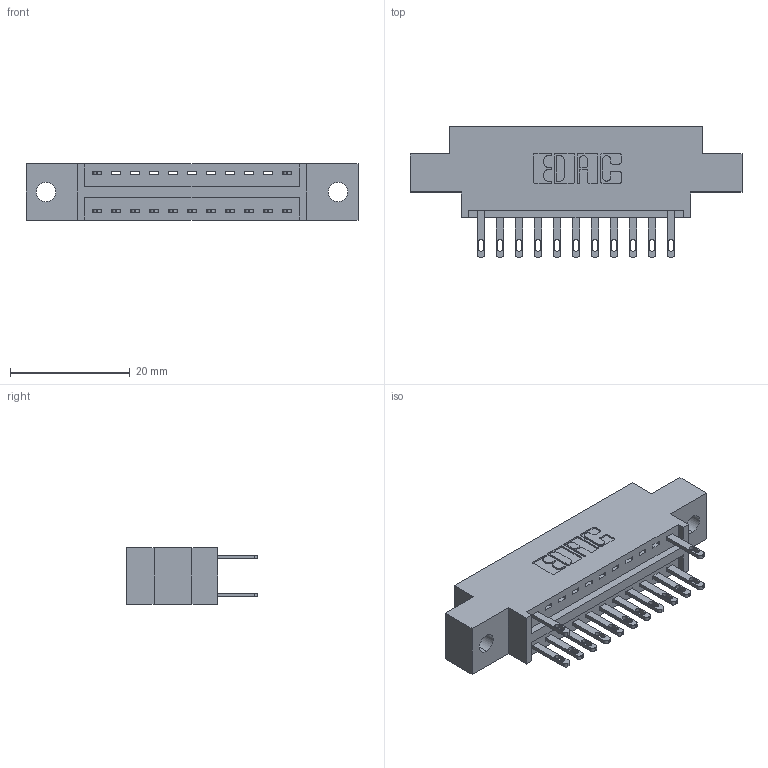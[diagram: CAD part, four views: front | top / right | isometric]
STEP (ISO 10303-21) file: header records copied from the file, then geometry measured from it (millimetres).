
FILE_DESCRIPTION (( 'STEP AP203' ), '1' );
FILE_NAME ('346-022-500-802.STEP', '2018-08-20T23:35:04', ( '' ), ( '' ), 'SwSTEP 2.0', 'SolidWorks 2016', '' );
FILE_SCHEMA (( 'CONFIG_CONTROL_DESIGN' ));
Length unit declared in the file: inch
Products named in the file (3): 345-292-001_345-293-100; 346-022-500-802; 346 Part_0.170 Offset - 0.128 Dia
Assembly tree (14 placements, depth 2):
  346-022-500-802
    346 Part_0.170 Offset - 0.128 Dia
    345-292-001_345-293-100  x13
Bounding box: 55.5 x 21.84 x 9.4 mm (x, y, z)
Volume: 4938.5 mm3; surface area: 5880.4 mm2
Topology: 14 solids, 14 shells, 804 faces, 2441 edges, 1626 vertices
Faces by surface type: plane 502, cylinder 302
Entity records: 11129 total; most frequent: CARTESIAN_POINT 1915, ORIENTED_EDGE 1858, DIRECTION 1731, EDGE_CURVE 929, LINE 749, VECTOR 749, VERTEX_POINT 618, AXIS2_PLACEMENT_3D 491
